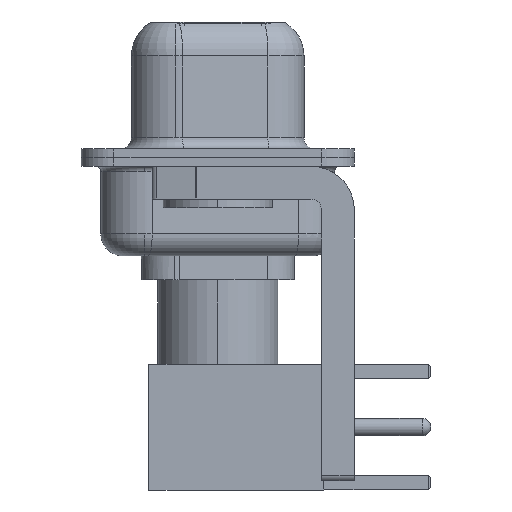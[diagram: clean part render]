
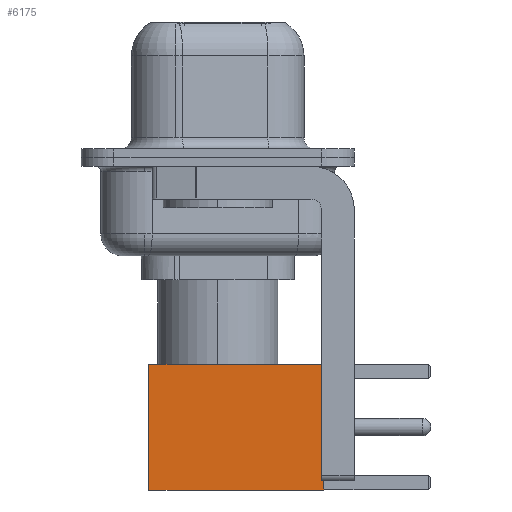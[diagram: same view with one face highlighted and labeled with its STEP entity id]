
A CAD part, left-side view. The second image highlights one B-rep face of the part: STEP entity #6175.
In plain terms, the highlighted face is planar.
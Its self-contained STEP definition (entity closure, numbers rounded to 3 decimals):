
#911 = EDGE_LOOP ( 'NONE', ( #8983, #14081, #12513, #7658 ) ) ;
#2603 = VERTEX_POINT ( 'NONE', #3199 ) ;
#3199 = CARTESIAN_POINT ( 'NONE',  ( 2.875, 2.875, 0. ) ) ;
#5077 = CARTESIAN_POINT ( 'NONE',  ( -2.875, 2.875, 0. ) ) ;
#5135 = DIRECTION ( 'NONE',  ( -1., 0., 0. ) ) ;
#5178 = DIRECTION ( 'NONE',  ( 0., 0., -1. ) ) ;
#6175 = ADVANCED_FACE ( 'NONE', ( #16660 ), #9297, .T. ) ;
#6575 = VERTEX_POINT ( 'NONE', #19876 ) ;
#7658 = ORIENTED_EDGE ( 'NONE', *, *, #14464, .F. ) ;
#7793 = CARTESIAN_POINT ( 'NONE',  ( 2.875, 2.875, 0. ) ) ;
#8072 = VERTEX_POINT ( 'NONE', #15305 ) ;
#8178 = LINE ( 'NONE', #15816, #12727 ) ;
#8233 = VERTEX_POINT ( 'NONE', #12582 ) ;
#8983 = ORIENTED_EDGE ( 'NONE', *, *, #19118, .T. ) ;
#9297 = PLANE ( 'NONE',  #10335 ) ;
#9890 = VECTOR ( 'NONE', #13529, 1000. ) ;
#10164 = LINE ( 'NONE', #16115, #10476 ) ;
#10335 = AXIS2_PLACEMENT_3D ( 'NONE', #7793, #15429, #19608 ) ;
#10454 = EDGE_CURVE ( 'NONE', #8072, #8233, #19011, .T. ) ;
#10476 = VECTOR ( 'NONE', #17834, 1000. ) ;
#12513 = ORIENTED_EDGE ( 'NONE', *, *, #10454, .F. ) ;
#12582 = CARTESIAN_POINT ( 'NONE',  ( -2.875, 2.875, 0. ) ) ;
#12727 = VECTOR ( 'NONE', #5135, 1000. ) ;
#13282 = VECTOR ( 'NONE', #5178, 1000. ) ;
#13529 = DIRECTION ( 'NONE',  ( 0., 0., -1. ) ) ;
#14081 = ORIENTED_EDGE ( 'NONE', *, *, #15771, .T. ) ;
#14464 = EDGE_CURVE ( 'NONE', #6575, #8072, #8178, .T. ) ;
#14635 = CARTESIAN_POINT ( 'NONE',  ( 2.875, 2.875, 0. ) ) ;
#14939 = LINE ( 'NONE', #14635, #9890 ) ;
#15305 = CARTESIAN_POINT ( 'NONE',  ( -2.875, 2.875, 8. ) ) ;
#15429 = DIRECTION ( 'NONE',  ( 0., 1., 0. ) ) ;
#15771 = EDGE_CURVE ( 'NONE', #2603, #8233, #10164, .T. ) ;
#15816 = CARTESIAN_POINT ( 'NONE',  ( 0., 2.875, 8. ) ) ;
#16115 = CARTESIAN_POINT ( 'NONE',  ( 0., 2.875, 0. ) ) ;
#16660 = FACE_OUTER_BOUND ( 'NONE', #911, .T. ) ;
#17834 = DIRECTION ( 'NONE',  ( -1., 0., 0. ) ) ;
#19011 = LINE ( 'NONE', #5077, #13282 ) ;
#19118 = EDGE_CURVE ( 'NONE', #6575, #2603, #14939, .T. ) ;
#19608 = DIRECTION ( 'NONE',  ( 0., 0., 1. ) ) ;
#19876 = CARTESIAN_POINT ( 'NONE',  ( 2.875, 2.875, 8. ) ) ;
